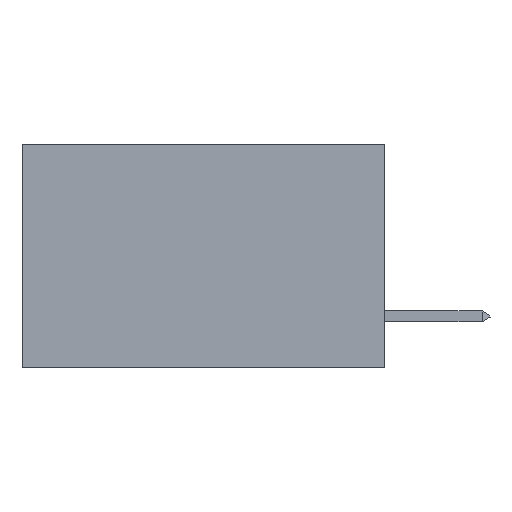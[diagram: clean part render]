
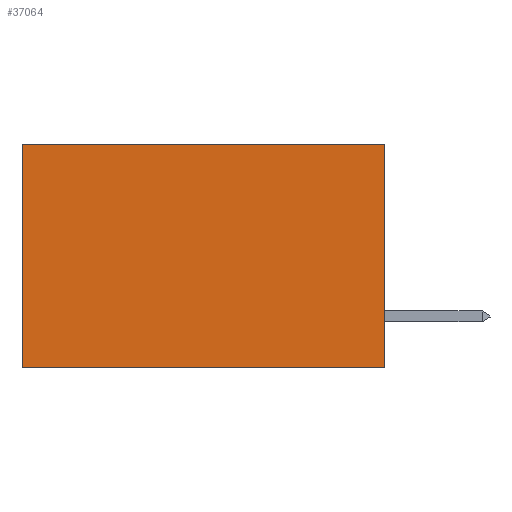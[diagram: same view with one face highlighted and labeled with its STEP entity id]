
A CAD part, left-side view. The second image highlights one B-rep face of the part: STEP entity #37064.
In plain terms, the highlighted planar face has unit normal (-1, 0, 0).
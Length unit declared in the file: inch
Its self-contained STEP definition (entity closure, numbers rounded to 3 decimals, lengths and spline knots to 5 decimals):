
#1389 = CARTESIAN_POINT ( 'NONE',  ( 0.2875, 0., 0. ) ) ;
#2545 = LINE ( 'NONE', #38026, #10692 ) ;
#3409 = ORIENTED_EDGE ( 'NONE', *, *, #13572, .F. ) ;
#6660 = CARTESIAN_POINT ( 'NONE',  ( 0.2875, 0.6, 0. ) ) ;
#7071 = VERTEX_POINT ( 'NONE', #32000 ) ;
#9805 = CARTESIAN_POINT ( 'NONE',  ( 0.2875, 0., -0.37 ) ) ;
#9894 = ORIENTED_EDGE ( 'NONE', *, *, #15335, .T. ) ;
#10692 = VECTOR ( 'NONE', #15257, 39.37008 ) ;
#10937 = ORIENTED_EDGE ( 'NONE', *, *, #18867, .T. ) ;
#11499 = LINE ( 'NONE', #6660, #22603 ) ;
#11735 = CARTESIAN_POINT ( 'NONE',  ( 0.2875, 0.6, -0.37 ) ) ;
#13011 = AXIS2_PLACEMENT_3D ( 'NONE', #24775, #21672, #21540 ) ;
#13325 = VERTEX_POINT ( 'NONE', #18397 ) ;
#13572 = EDGE_CURVE ( 'NONE', #18452, #30011, #25287, .T. ) ;
#13997 = CARTESIAN_POINT ( 'NONE',  ( 0.2875, 0., -0.37 ) ) ;
#15257 = DIRECTION ( 'NONE',  ( 0., 1., 0. ) ) ;
#15335 = EDGE_CURVE ( 'NONE', #13325, #30011, #11499, .T. ) ;
#18397 = CARTESIAN_POINT ( 'NONE',  ( 0.2875, 0.6, 0. ) ) ;
#18452 = VERTEX_POINT ( 'NONE', #9805 ) ;
#18867 = EDGE_CURVE ( 'NONE', #7071, #13325, #2545, .T. ) ;
#20302 = EDGE_CURVE ( 'NONE', #7071, #18452, #33344, .T. ) ;
#21540 = DIRECTION ( 'NONE',  ( 0., 0., -1. ) ) ;
#21672 = DIRECTION ( 'NONE',  ( 1., 0., 0. ) ) ;
#22603 = VECTOR ( 'NONE', #29022, 39.37008 ) ;
#23788 = VECTOR ( 'NONE', #39619, 39.37008 ) ;
#24775 = CARTESIAN_POINT ( 'NONE',  ( 0.2875, 0., 0. ) ) ;
#25287 = LINE ( 'NONE', #13997, #23788 ) ;
#29022 = DIRECTION ( 'NONE',  ( 0., 0., -1. ) ) ;
#30011 = VERTEX_POINT ( 'NONE', #11735 ) ;
#30830 = DIRECTION ( 'NONE',  ( 0., 0., -1. ) ) ;
#32000 = CARTESIAN_POINT ( 'NONE',  ( 0.2875, 0., 0. ) ) ;
#32332 = VECTOR ( 'NONE', #30830, 39.37008 ) ;
#33344 = LINE ( 'NONE', #1389, #32332 ) ;
#37064 = ADVANCED_FACE ( 'NONE', ( #37214 ), #37789, .F. ) ;
#37214 = FACE_OUTER_BOUND ( 'NONE', #40763, .T. ) ;
#37789 = PLANE ( 'NONE',  #13011 ) ;
#38026 = CARTESIAN_POINT ( 'NONE',  ( 0.2875, 0., 0. ) ) ;
#38571 = ORIENTED_EDGE ( 'NONE', *, *, #20302, .F. ) ;
#39619 = DIRECTION ( 'NONE',  ( 0., 1., 0. ) ) ;
#40763 = EDGE_LOOP ( 'NONE', ( #9894, #3409, #38571, #10937 ) ) ;
